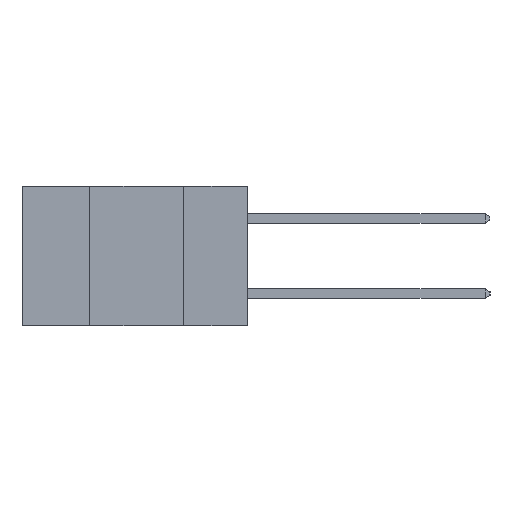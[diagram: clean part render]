
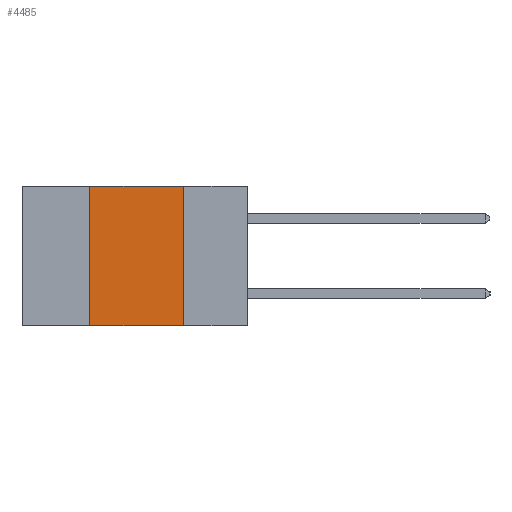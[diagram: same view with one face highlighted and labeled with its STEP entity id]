
A CAD part, left-side view. The second image highlights one B-rep face of the part: STEP entity #4485.
In plain terms, the highlighted planar face has unit normal (-1, 0, 0).
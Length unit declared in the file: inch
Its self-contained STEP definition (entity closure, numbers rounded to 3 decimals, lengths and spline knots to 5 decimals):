
#146 = LINE ( 'NONE', #21080, #15129 ) ;
#364 = EDGE_CURVE ( 'NONE', #15599, #2997, #146, .T. ) ;
#496 = ORIENTED_EDGE ( 'NONE', *, *, #8378, .F. ) ;
#1022 = LINE ( 'NONE', #14095, #4991 ) ;
#1023 = ORIENTED_EDGE ( 'NONE', *, *, #20935, .F. ) ;
#1227 = LINE ( 'NONE', #16145, #12741 ) ;
#1305 = VERTEX_POINT ( 'NONE', #3919 ) ;
#1732 = AXIS2_PLACEMENT_3D ( 'NONE', #5247, #4795, #3463 ) ;
#2997 = VERTEX_POINT ( 'NONE', #14819 ) ;
#3284 = VECTOR ( 'NONE', #17018, 39.37008 ) ;
#3463 = DIRECTION ( 'NONE',  ( 0., 0., -1. ) ) ;
#3919 = CARTESIAN_POINT ( 'NONE',  ( 0., 0.17, 0. ) ) ;
#4485 = ADVANCED_FACE ( 'NONE', ( #17193 ), #10317, .F. ) ;
#4795 = DIRECTION ( 'NONE',  ( 1., 0., 0. ) ) ;
#4906 = CARTESIAN_POINT ( 'NONE',  ( 0., 0.42, 0. ) ) ;
#4991 = VECTOR ( 'NONE', #19621, 39.37008 ) ;
#5247 = CARTESIAN_POINT ( 'NONE',  ( 0., 0.6, 0. ) ) ;
#5883 = CARTESIAN_POINT ( 'NONE',  ( 0., 0.42, -0.37 ) ) ;
#5920 = EDGE_LOOP ( 'NONE', ( #9044, #496, #1023, #14682 ) ) ;
#6753 = CARTESIAN_POINT ( 'NONE',  ( 0., 0.42, -0.37 ) ) ;
#8378 = EDGE_CURVE ( 'NONE', #16248, #1305, #1022, .T. ) ;
#9044 = ORIENTED_EDGE ( 'NONE', *, *, #15262, .F. ) ;
#10317 = PLANE ( 'NONE',  #1732 ) ;
#12693 = DIRECTION ( 'NONE',  ( 0., 0., -1. ) ) ;
#12741 = VECTOR ( 'NONE', #12693, 39.37008 ) ;
#13495 = LINE ( 'NONE', #5883, #3284 ) ;
#14095 = CARTESIAN_POINT ( 'NONE',  ( 0., 0.6, 0. ) ) ;
#14682 = ORIENTED_EDGE ( 'NONE', *, *, #364, .T. ) ;
#14819 = CARTESIAN_POINT ( 'NONE',  ( 0., 0.17, -0.37 ) ) ;
#15129 = VECTOR ( 'NONE', #21175, 39.37008 ) ;
#15262 = EDGE_CURVE ( 'NONE', #1305, #2997, #1227, .T. ) ;
#15599 = VERTEX_POINT ( 'NONE', #6753 ) ;
#16145 = CARTESIAN_POINT ( 'NONE',  ( 0., 0.17, -0.37 ) ) ;
#16248 = VERTEX_POINT ( 'NONE', #4906 ) ;
#17018 = DIRECTION ( 'NONE',  ( 0., 0., 1. ) ) ;
#17193 = FACE_OUTER_BOUND ( 'NONE', #5920, .T. ) ;
#19621 = DIRECTION ( 'NONE',  ( 0., -1., 0. ) ) ;
#20935 = EDGE_CURVE ( 'NONE', #15599, #16248, #13495, .T. ) ;
#21080 = CARTESIAN_POINT ( 'NONE',  ( 0., 0.6, -0.37 ) ) ;
#21175 = DIRECTION ( 'NONE',  ( 0., -1., 0. ) ) ;
